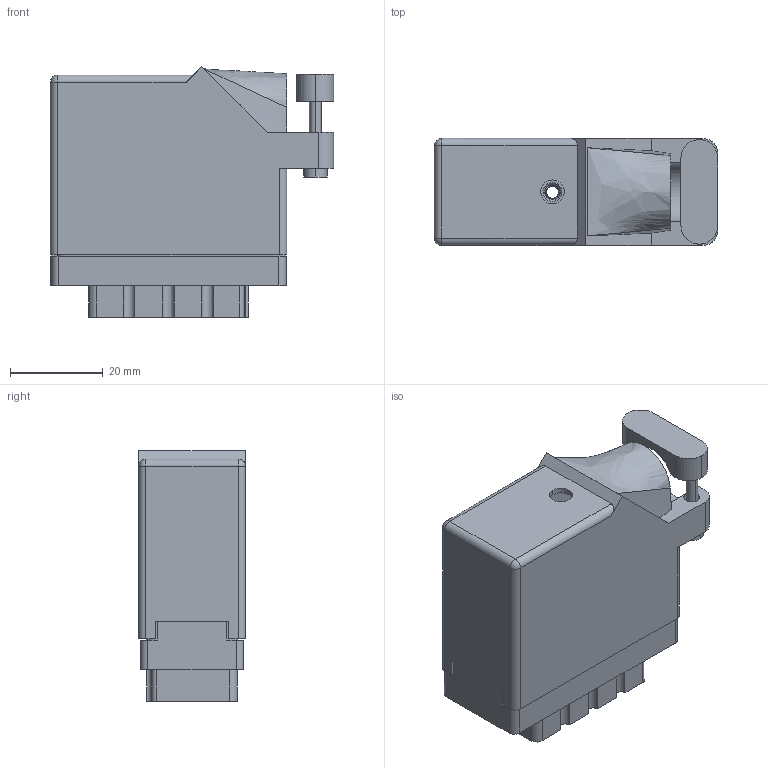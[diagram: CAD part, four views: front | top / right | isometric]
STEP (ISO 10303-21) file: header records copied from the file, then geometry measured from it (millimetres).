
FILE_DESCRIPTION (( 'STEP AP203' ), '1' );
FILE_NAME ('516-038-000-226.STEP', '2020-03-04T21:23:37', ( '' ), ( '' ), 'SwSTEP 2.0', 'SolidWorks 2016', '' );
FILE_SCHEMA (( 'CONFIG_CONTROL_DESIGN' ));
Length unit declared in the file: inch
Products named in the file (4): 516-230-001_Plastic - 038 Side Entry; 516-038-000-226; 516-252-035-100_516-252-035-100; 516 Part Receptacle_038
Assembly tree (3 placements, depth 2):
  516-038-000-226
    516 Part Receptacle_038
    516-230-001_Plastic - 038 Side Entry
    516-252-035-100_516-252-035-100
Bounding box: 61.21 x 23.11 x 54.15 mm (x, y, z)
Volume: 21347.1 mm3; surface area: 28925.1 mm2
Topology: 3 solids, 3 shells, 1041 faces, 3022 edges, 2008 vertices
Faces by surface type: plane 685, cylinder 333, cone 12, bspline 9, sphere 2
Entity records: 37334 total; most frequent: CARTESIAN_POINT 8614, ORIENTED_EDGE 6040, DIRECTION 5848, EDGE_CURVE 3020, VECTOR 2160, LINE 2160, VERTEX_POINT 2008, AXIS2_PLACEMENT_3D 1844
